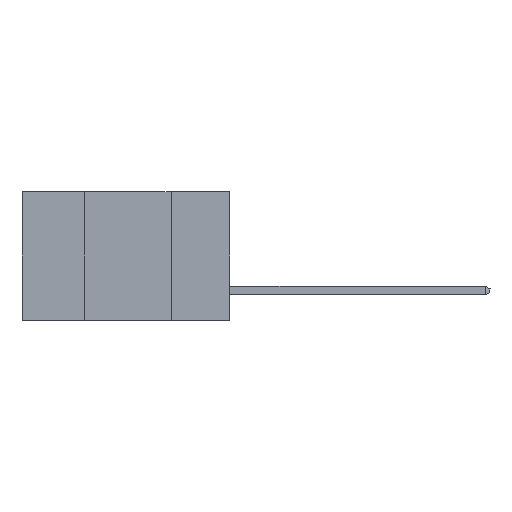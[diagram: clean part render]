
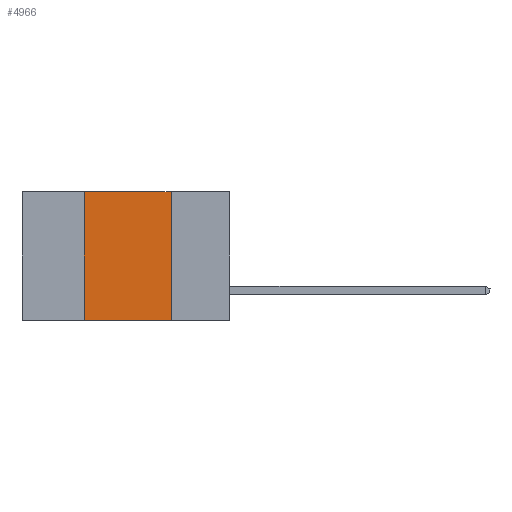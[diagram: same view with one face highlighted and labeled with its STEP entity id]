
A CAD part, left-side view. The second image highlights one B-rep face of the part: STEP entity #4966.
In plain terms, the highlighted planar face has unit normal (-1, 0, 0).
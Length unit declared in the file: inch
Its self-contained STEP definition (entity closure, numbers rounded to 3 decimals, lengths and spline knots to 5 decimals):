
#126 = CARTESIAN_POINT ( 'NONE',  ( 0., 0.6, 0. ) ) ;
#324 = EDGE_CURVE ( 'NONE', #4407, #2773, #2676, .T. ) ;
#511 = CARTESIAN_POINT ( 'NONE',  ( 0., 0.6, 0. ) ) ;
#1017 = ORIENTED_EDGE ( 'NONE', *, *, #324, .T. ) ;
#1099 = CARTESIAN_POINT ( 'NONE',  ( 0., 0.6, -0.37 ) ) ;
#1351 = DIRECTION ( 'NONE',  ( 0., -1., 0. ) ) ;
#2308 = VECTOR ( 'NONE', #8286, 39.37008 ) ;
#2507 = VECTOR ( 'NONE', #5377, 39.37008 ) ;
#2518 = CARTESIAN_POINT ( 'NONE',  ( 0., 0.42, -0.37 ) ) ;
#2525 = VECTOR ( 'NONE', #7832, 39.37008 ) ;
#2676 = LINE ( 'NONE', #1099, #2308 ) ;
#2773 = VERTEX_POINT ( 'NONE', #5387 ) ;
#2974 = CARTESIAN_POINT ( 'NONE',  ( 0., 0.17, -0.37 ) ) ;
#3382 = EDGE_CURVE ( 'NONE', #8119, #4411, #9322, .T. ) ;
#4407 = VERTEX_POINT ( 'NONE', #6305 ) ;
#4411 = VERTEX_POINT ( 'NONE', #5508 ) ;
#4433 = CARTESIAN_POINT ( 'NONE',  ( 0., 0.42, 0. ) ) ;
#4605 = LINE ( 'NONE', #2974, #2525 ) ;
#4941 = ORIENTED_EDGE ( 'NONE', *, *, #9233, .F. ) ;
#4966 = ADVANCED_FACE ( 'NONE', ( #9731 ), #9630, .F. ) ;
#5377 = DIRECTION ( 'NONE',  ( 0., 0., 1. ) ) ;
#5387 = CARTESIAN_POINT ( 'NONE',  ( 0., 0.17, -0.37 ) ) ;
#5508 = CARTESIAN_POINT ( 'NONE',  ( 0., 0.17, 0. ) ) ;
#5602 = AXIS2_PLACEMENT_3D ( 'NONE', #126, #8200, #8820 ) ;
#6217 = LINE ( 'NONE', #2518, #2507 ) ;
#6305 = CARTESIAN_POINT ( 'NONE',  ( 0., 0.42, -0.37 ) ) ;
#7832 = DIRECTION ( 'NONE',  ( 0., 0., -1. ) ) ;
#8119 = VERTEX_POINT ( 'NONE', #4433 ) ;
#8200 = DIRECTION ( 'NONE',  ( 1., 0., 0. ) ) ;
#8286 = DIRECTION ( 'NONE',  ( 0., -1., 0. ) ) ;
#8499 = ORIENTED_EDGE ( 'NONE', *, *, #9978, .F. ) ;
#8820 = DIRECTION ( 'NONE',  ( 0., 0., -1. ) ) ;
#8846 = EDGE_LOOP ( 'NONE', ( #8499, #9743, #4941, #1017 ) ) ;
#9233 = EDGE_CURVE ( 'NONE', #4407, #8119, #6217, .T. ) ;
#9322 = LINE ( 'NONE', #511, #9324 ) ;
#9324 = VECTOR ( 'NONE', #1351, 39.37008 ) ;
#9630 = PLANE ( 'NONE',  #5602 ) ;
#9731 = FACE_OUTER_BOUND ( 'NONE', #8846, .T. ) ;
#9743 = ORIENTED_EDGE ( 'NONE', *, *, #3382, .F. ) ;
#9978 = EDGE_CURVE ( 'NONE', #4411, #2773, #4605, .T. ) ;
